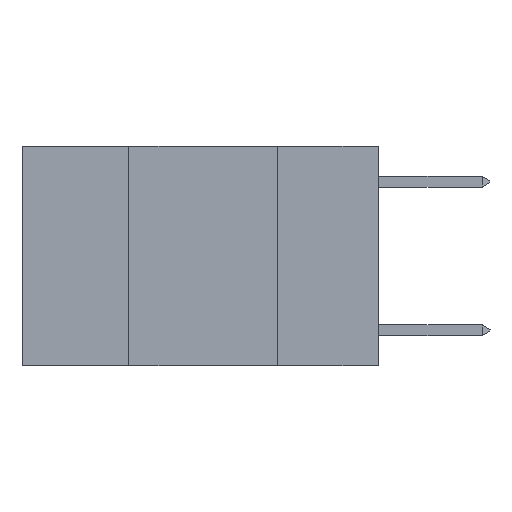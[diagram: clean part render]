
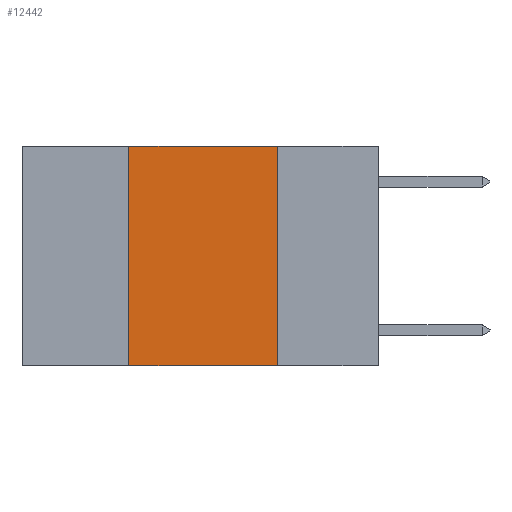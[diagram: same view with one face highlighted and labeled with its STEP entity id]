
A CAD part, left-side view. The second image highlights one B-rep face of the part: STEP entity #12442.
In plain terms, the highlighted planar face has unit normal (-1, 0, 0).
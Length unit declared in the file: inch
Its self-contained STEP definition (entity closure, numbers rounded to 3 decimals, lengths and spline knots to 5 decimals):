
#73 = VERTEX_POINT ( 'NONE', #6369 ) ;
#425 = VERTEX_POINT ( 'NONE', #8693 ) ;
#881 = DIRECTION ( 'NONE',  ( 0., -1., 0. ) ) ;
#1336 = VERTEX_POINT ( 'NONE', #3316 ) ;
#2358 = EDGE_LOOP ( 'NONE', ( #7507, #7588, #7663, #7767 ) ) ;
#2767 = CARTESIAN_POINT ( 'NONE',  ( 0., 0.6, 0. ) ) ;
#2881 = VECTOR ( 'NONE', #3816, 39.37008 ) ;
#3316 = CARTESIAN_POINT ( 'NONE',  ( 0., 0.17, -0.37 ) ) ;
#3434 = DIRECTION ( 'NONE',  ( 0., -1., 0. ) ) ;
#3816 = DIRECTION ( 'NONE',  ( 0., 0., -1. ) ) ;
#4010 = CARTESIAN_POINT ( 'NONE',  ( 0., 0.6, -0.37 ) ) ;
#4710 = FACE_OUTER_BOUND ( 'NONE', #2358, .T. ) ;
#4807 = DIRECTION ( 'NONE',  ( 0., 0., -1. ) ) ;
#4837 = CARTESIAN_POINT ( 'NONE',  ( 0., 0.17, 0. ) ) ;
#5082 = LINE ( 'NONE', #9836, #12634 ) ;
#6369 = CARTESIAN_POINT ( 'NONE',  ( 0., 0.42, -0.37 ) ) ;
#6433 = LINE ( 'NONE', #12348, #9098 ) ;
#6676 = EDGE_CURVE ( 'NONE', #425, #7524, #6433, .T. ) ;
#7507 = ORIENTED_EDGE ( 'NONE', *, *, #10106, .F. ) ;
#7524 = VERTEX_POINT ( 'NONE', #4837 ) ;
#7588 = ORIENTED_EDGE ( 'NONE', *, *, #6676, .F. ) ;
#7663 = ORIENTED_EDGE ( 'NONE', *, *, #10760, .F. ) ;
#7767 = ORIENTED_EDGE ( 'NONE', *, *, #12696, .T. ) ;
#8693 = CARTESIAN_POINT ( 'NONE',  ( 0., 0.42, 0. ) ) ;
#8706 = AXIS2_PLACEMENT_3D ( 'NONE', #2767, #10748, #4807 ) ;
#9098 = VECTOR ( 'NONE', #3434, 39.37008 ) ;
#9545 = VECTOR ( 'NONE', #881, 39.37008 ) ;
#9764 = PLANE ( 'NONE',  #8706 ) ;
#9775 = CARTESIAN_POINT ( 'NONE',  ( 0., 0.17, 0. ) ) ;
#9836 = CARTESIAN_POINT ( 'NONE',  ( 0., 0.42, 0. ) ) ;
#10106 = EDGE_CURVE ( 'NONE', #7524, #1336, #10839, .T. ) ;
#10748 = DIRECTION ( 'NONE',  ( 1., 0., 0. ) ) ;
#10760 = EDGE_CURVE ( 'NONE', #73, #425, #5082, .T. ) ;
#10839 = LINE ( 'NONE', #9775, #2881 ) ;
#12129 = LINE ( 'NONE', #4010, #9545 ) ;
#12348 = CARTESIAN_POINT ( 'NONE',  ( 0., 0.6, 0. ) ) ;
#12442 = ADVANCED_FACE ( 'NONE', ( #4710 ), #9764, .F. ) ;
#12634 = VECTOR ( 'NONE', #12771, 39.37008 ) ;
#12696 = EDGE_CURVE ( 'NONE', #73, #1336, #12129, .T. ) ;
#12771 = DIRECTION ( 'NONE',  ( 0., 0., 1. ) ) ;
